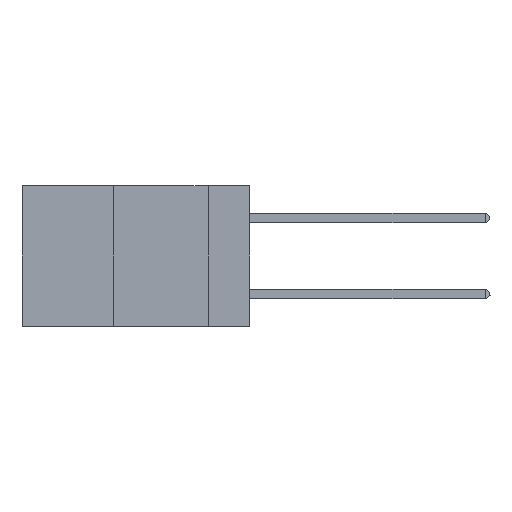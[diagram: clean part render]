
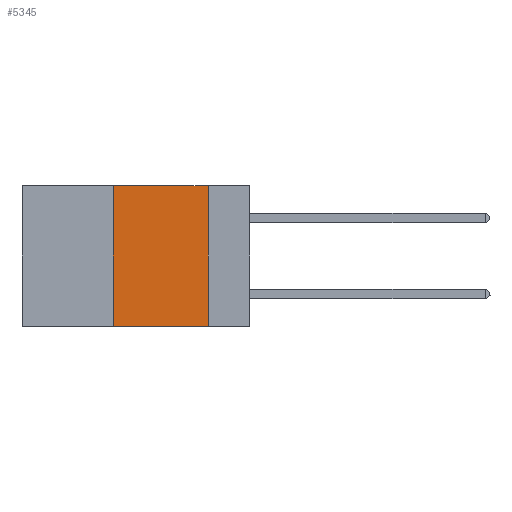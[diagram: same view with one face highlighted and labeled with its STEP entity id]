
A CAD part, left-side view. The second image highlights one B-rep face of the part: STEP entity #5345.
In plain terms, the highlighted planar face has unit normal (-1, 0, 0).
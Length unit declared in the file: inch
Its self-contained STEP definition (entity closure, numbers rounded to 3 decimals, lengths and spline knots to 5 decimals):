
#477 = CARTESIAN_POINT ( 'NONE',  ( 0., 0.36, -0.37 ) ) ;
#590 = DIRECTION ( 'NONE',  ( 1., 0., 0. ) ) ;
#656 = DIRECTION ( 'NONE',  ( 0., 0., -1. ) ) ;
#1792 = CARTESIAN_POINT ( 'NONE',  ( 0., 0.11, -0.37 ) ) ;
#2255 = LINE ( 'NONE', #10637, #6982 ) ;
#2892 = AXIS2_PLACEMENT_3D ( 'NONE', #7422, #590, #656 ) ;
#4072 = VECTOR ( 'NONE', #8684, 39.37008 ) ;
#4128 = ORIENTED_EDGE ( 'NONE', *, *, #11839, .F. ) ;
#5345 = ADVANCED_FACE ( 'NONE', ( #16425 ), #15701, .F. ) ;
#5355 = ORIENTED_EDGE ( 'NONE', *, *, #12319, .F. ) ;
#6160 = VECTOR ( 'NONE', #11619, 39.37008 ) ;
#6286 = VERTEX_POINT ( 'NONE', #1792 ) ;
#6300 = ORIENTED_EDGE ( 'NONE', *, *, #11206, .F. ) ;
#6982 = VECTOR ( 'NONE', #10929, 39.37008 ) ;
#7119 = LINE ( 'NONE', #8741, #4072 ) ;
#7226 = EDGE_LOOP ( 'NONE', ( #5355, #4128, #6300, #12990 ) ) ;
#7422 = CARTESIAN_POINT ( 'NONE',  ( 0., 0.6, 0. ) ) ;
#7772 = VERTEX_POINT ( 'NONE', #15515 ) ;
#8371 = EDGE_CURVE ( 'NONE', #15612, #6286, #7119, .T. ) ;
#8684 = DIRECTION ( 'NONE',  ( 0., -1., 0. ) ) ;
#8741 = CARTESIAN_POINT ( 'NONE',  ( 0., 0.6, -0.37 ) ) ;
#9663 = DIRECTION ( 'NONE',  ( 0., -1., 0. ) ) ;
#10227 = CARTESIAN_POINT ( 'NONE',  ( 0., 0.6, 0. ) ) ;
#10637 = CARTESIAN_POINT ( 'NONE',  ( 0., 0.36, 0. ) ) ;
#10929 = DIRECTION ( 'NONE',  ( 0., 0., 1. ) ) ;
#11206 = EDGE_CURVE ( 'NONE', #15612, #7772, #2255, .T. ) ;
#11619 = DIRECTION ( 'NONE',  ( 0., 0., -1. ) ) ;
#11627 = LINE ( 'NONE', #10227, #12257 ) ;
#11839 = EDGE_CURVE ( 'NONE', #7772, #11977, #11627, .T. ) ;
#11977 = VERTEX_POINT ( 'NONE', #14511 ) ;
#12257 = VECTOR ( 'NONE', #9663, 39.37008 ) ;
#12319 = EDGE_CURVE ( 'NONE', #11977, #6286, #14446, .T. ) ;
#12990 = ORIENTED_EDGE ( 'NONE', *, *, #8371, .T. ) ;
#14446 = LINE ( 'NONE', #15920, #6160 ) ;
#14511 = CARTESIAN_POINT ( 'NONE',  ( 0., 0.11, 0. ) ) ;
#15515 = CARTESIAN_POINT ( 'NONE',  ( 0., 0.36, 0. ) ) ;
#15612 = VERTEX_POINT ( 'NONE', #477 ) ;
#15701 = PLANE ( 'NONE',  #2892 ) ;
#15920 = CARTESIAN_POINT ( 'NONE',  ( 0., 0.11, 0. ) ) ;
#16425 = FACE_OUTER_BOUND ( 'NONE', #7226, .T. ) ;
